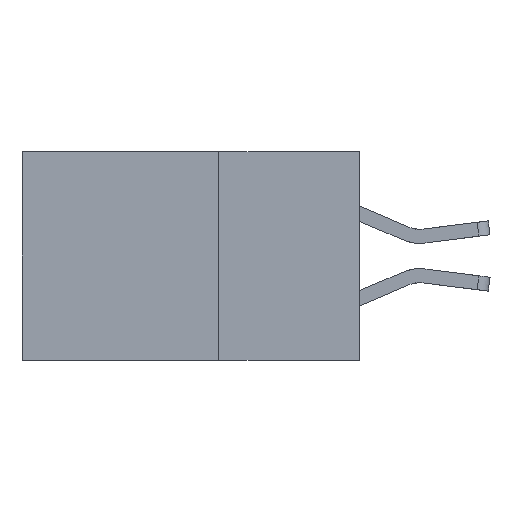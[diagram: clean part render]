
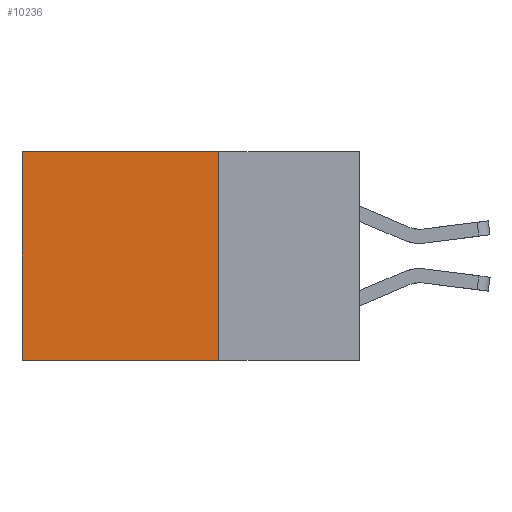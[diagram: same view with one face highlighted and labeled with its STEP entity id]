
A CAD part, left-side view. The second image highlights one B-rep face of the part: STEP entity #10236.
In plain terms, the highlighted planar face has unit normal (-1, 0, 0).
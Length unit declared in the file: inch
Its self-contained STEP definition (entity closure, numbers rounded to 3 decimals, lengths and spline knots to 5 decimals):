
#64 = CARTESIAN_POINT ( 'NONE',  ( 0.2875, 0.6, 0. ) ) ;
#593 = VERTEX_POINT ( 'NONE', #10545 ) ;
#917 = EDGE_LOOP ( 'NONE', ( #11681, #11503, #13579, #1511 ) ) ;
#1511 = ORIENTED_EDGE ( 'NONE', *, *, #3165, .T. ) ;
#1913 = CARTESIAN_POINT ( 'NONE',  ( 0.2875, 0.25, 0. ) ) ;
#2155 = VERTEX_POINT ( 'NONE', #6163 ) ;
#2218 = CARTESIAN_POINT ( 'NONE',  ( 0.2875, 0.25, -0.37 ) ) ;
#2334 = DIRECTION ( 'NONE',  ( 0., 1., 0. ) ) ;
#2421 = VERTEX_POINT ( 'NONE', #4009 ) ;
#2573 = VECTOR ( 'NONE', #10740, 39.37008 ) ;
#3165 = EDGE_CURVE ( 'NONE', #2421, #593, #4966, .T. ) ;
#3663 = DIRECTION ( 'NONE',  ( 0., 0., -1. ) ) ;
#3920 = LINE ( 'NONE', #2218, #6534 ) ;
#4009 = CARTESIAN_POINT ( 'NONE',  ( 0.2875, 0.25, 0. ) ) ;
#4122 = FACE_OUTER_BOUND ( 'NONE', #917, .T. ) ;
#4678 = DIRECTION ( 'NONE',  ( 0., 0., -1. ) ) ;
#4966 = LINE ( 'NONE', #7881, #7542 ) ;
#6163 = CARTESIAN_POINT ( 'NONE',  ( 0.2875, 0.25, -0.37 ) ) ;
#6534 = VECTOR ( 'NONE', #13194, 39.37008 ) ;
#6928 = VECTOR ( 'NONE', #4678, 39.37008 ) ;
#6982 = PLANE ( 'NONE',  #9366 ) ;
#7158 = EDGE_CURVE ( 'NONE', #2421, #2155, #13839, .T. ) ;
#7464 = EDGE_CURVE ( 'NONE', #593, #11996, #9814, .T. ) ;
#7542 = VECTOR ( 'NONE', #2334, 39.37008 ) ;
#7881 = CARTESIAN_POINT ( 'NONE',  ( 0.2875, 0.25, 0. ) ) ;
#9068 = CARTESIAN_POINT ( 'NONE',  ( 0.2875, 0.6, -0.37 ) ) ;
#9366 = AXIS2_PLACEMENT_3D ( 'NONE', #13440, #10251, #3663 ) ;
#9814 = LINE ( 'NONE', #64, #6928 ) ;
#10236 = ADVANCED_FACE ( 'NONE', ( #4122 ), #6982, .F. ) ;
#10251 = DIRECTION ( 'NONE',  ( 1., 0., 0. ) ) ;
#10545 = CARTESIAN_POINT ( 'NONE',  ( 0.2875, 0.6, 0. ) ) ;
#10740 = DIRECTION ( 'NONE',  ( 0., 0., -1. ) ) ;
#11503 = ORIENTED_EDGE ( 'NONE', *, *, #12458, .F. ) ;
#11681 = ORIENTED_EDGE ( 'NONE', *, *, #7464, .T. ) ;
#11996 = VERTEX_POINT ( 'NONE', #9068 ) ;
#12458 = EDGE_CURVE ( 'NONE', #2155, #11996, #3920, .T. ) ;
#13194 = DIRECTION ( 'NONE',  ( 0., 1., 0. ) ) ;
#13440 = CARTESIAN_POINT ( 'NONE',  ( 0.2875, 0.25, 0. ) ) ;
#13579 = ORIENTED_EDGE ( 'NONE', *, *, #7158, .F. ) ;
#13839 = LINE ( 'NONE', #1913, #2573 ) ;
